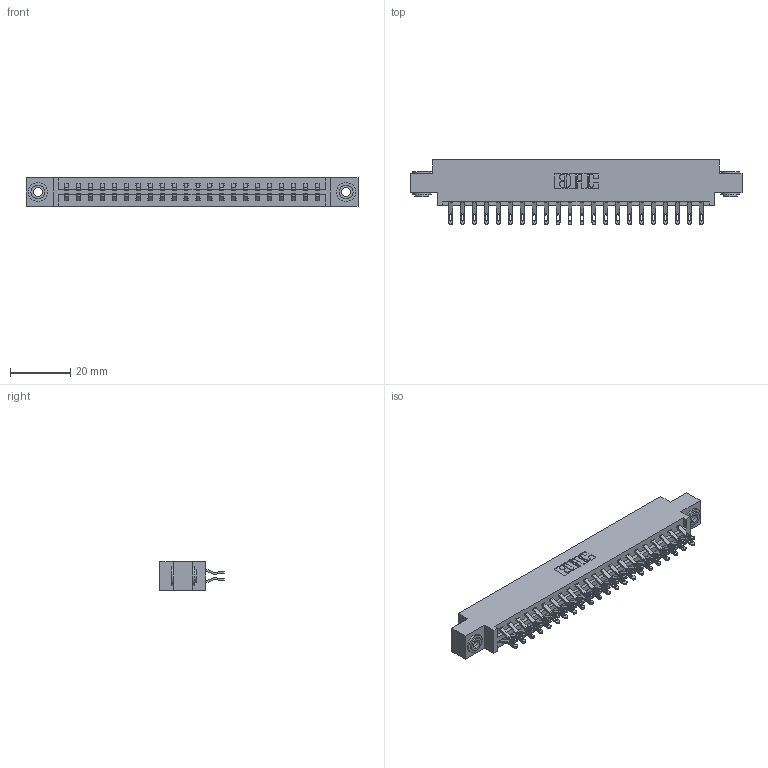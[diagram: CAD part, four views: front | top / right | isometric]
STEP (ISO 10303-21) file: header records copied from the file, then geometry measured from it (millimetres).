
FILE_DESCRIPTION (( 'STEP AP203' ), '1' );
FILE_NAME ('387-044-555-803.STEP', '2018-09-20T02:40:27', ( '' ), ( '' ), 'SwSTEP 2.0', 'SolidWorks 2016', '' );
FILE_SCHEMA (( 'CONFIG_CONTROL_DESIGN' ));
Length unit declared in the file: inch
Products named in the file (4): 337 Part_0.170 Offset - 0.156 Dia-TH; 345-292-001_555 Tail; 345-250-002_345-250-002-102; 387-044-555-803
Assembly tree (47 placements, depth 2):
  387-044-555-803
    337 Part_0.170 Offset - 0.156 Dia-TH
    345-292-001_555 Tail  x44
    345-250-002_345-250-002-102  x2
Bounding box: 110.19 x 21.47 x 9.4 mm (x, y, z)
Volume: 11375.5 mm3; surface area: 13478.9 mm2
Topology: 47 solids, 47 shells, 2796 faces, 8715 edges, 5806 vertices
Faces by surface type: plane 1668, cylinder 1120, cone 8
Entity records: 20752 total; most frequent: CARTESIAN_POINT 3523, ORIENTED_EDGE 3422, DIRECTION 3037, EDGE_CURVE 1711, VECTOR 1539, LINE 1539, VERTEX_POINT 1138, AXIS2_PLACEMENT_3D 749
